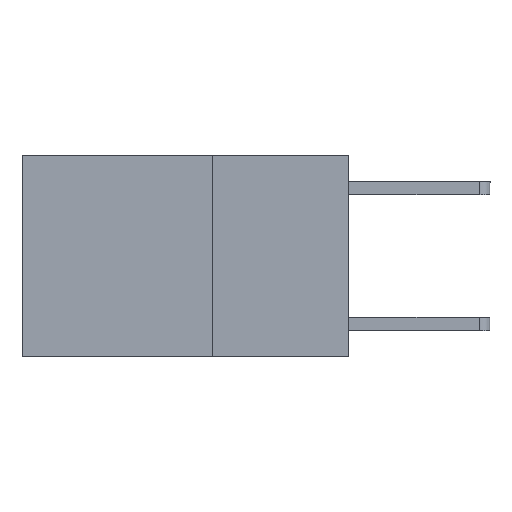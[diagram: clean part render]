
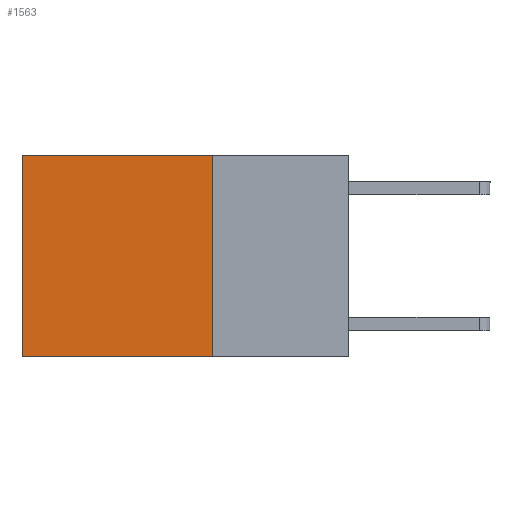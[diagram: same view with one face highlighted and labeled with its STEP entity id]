
A CAD part, left-side view. The second image highlights one B-rep face of the part: STEP entity #1563.
In plain terms, the highlighted planar face has unit normal (-1, 0, 0).
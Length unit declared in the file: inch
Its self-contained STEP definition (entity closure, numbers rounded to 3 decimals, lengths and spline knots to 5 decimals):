
#292 = EDGE_CURVE ( 'NONE', #2937, #1504, #5560, .T. ) ;
#563 = CARTESIAN_POINT ( 'NONE',  ( 0.2625, 0.6, 0. ) ) ;
#610 = VECTOR ( 'NONE', #5176, 39.37008 ) ;
#969 = DIRECTION ( 'NONE',  ( 0., 0., -1. ) ) ;
#1294 = ORIENTED_EDGE ( 'NONE', *, *, #1518, .T. ) ;
#1473 = CARTESIAN_POINT ( 'NONE',  ( 0.2625, 0.25, -0.37 ) ) ;
#1504 = VERTEX_POINT ( 'NONE', #4655 ) ;
#1518 = EDGE_CURVE ( 'NONE', #1881, #8191, #4831, .T. ) ;
#1563 = ADVANCED_FACE ( 'NONE', ( #2960 ), #4226, .F. ) ;
#1577 = DIRECTION ( 'NONE',  ( 0., 1., 0. ) ) ;
#1656 = CARTESIAN_POINT ( 'NONE',  ( 0.2625, 0.25, 0. ) ) ;
#1668 = CARTESIAN_POINT ( 'NONE',  ( 0.2625, 0.25, -0.37 ) ) ;
#1735 = LINE ( 'NONE', #1656, #3022 ) ;
#1881 = VERTEX_POINT ( 'NONE', #8182 ) ;
#2937 = VERTEX_POINT ( 'NONE', #1473 ) ;
#2960 = FACE_OUTER_BOUND ( 'NONE', #6795, .T. ) ;
#2999 = ORIENTED_EDGE ( 'NONE', *, *, #292, .F. ) ;
#3022 = VECTOR ( 'NONE', #6324, 39.37008 ) ;
#3161 = ORIENTED_EDGE ( 'NONE', *, *, #5152, .F. ) ;
#3703 = AXIS2_PLACEMENT_3D ( 'NONE', #4912, #8345, #969 ) ;
#3781 = EDGE_CURVE ( 'NONE', #8191, #1504, #7741, .T. ) ;
#4180 = CARTESIAN_POINT ( 'NONE',  ( 0.2625, 0.25, 0. ) ) ;
#4226 = PLANE ( 'NONE',  #3703 ) ;
#4622 = VECTOR ( 'NONE', #1577, 39.37008 ) ;
#4655 = CARTESIAN_POINT ( 'NONE',  ( 0.2625, 0.6, -0.37 ) ) ;
#4831 = LINE ( 'NONE', #4180, #4942 ) ;
#4912 = CARTESIAN_POINT ( 'NONE',  ( 0.2625, 0.25, 0. ) ) ;
#4942 = VECTOR ( 'NONE', #6826, 39.37008 ) ;
#5152 = EDGE_CURVE ( 'NONE', #1881, #2937, #1735, .T. ) ;
#5176 = DIRECTION ( 'NONE',  ( 0., 0., -1. ) ) ;
#5560 = LINE ( 'NONE', #1668, #4622 ) ;
#6324 = DIRECTION ( 'NONE',  ( 0., 0., -1. ) ) ;
#6795 = EDGE_LOOP ( 'NONE', ( #7442, #2999, #3161, #1294 ) ) ;
#6826 = DIRECTION ( 'NONE',  ( 0., 1., 0. ) ) ;
#7442 = ORIENTED_EDGE ( 'NONE', *, *, #3781, .T. ) ;
#7741 = LINE ( 'NONE', #563, #610 ) ;
#8182 = CARTESIAN_POINT ( 'NONE',  ( 0.2625, 0.25, 0. ) ) ;
#8191 = VERTEX_POINT ( 'NONE', #8238 ) ;
#8238 = CARTESIAN_POINT ( 'NONE',  ( 0.2625, 0.6, 0. ) ) ;
#8345 = DIRECTION ( 'NONE',  ( 1., 0., 0. ) ) ;
